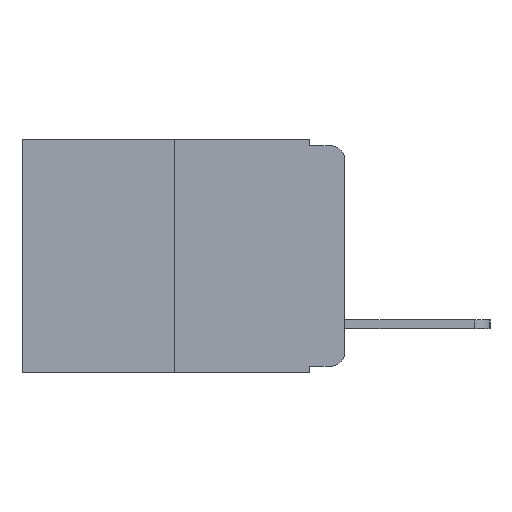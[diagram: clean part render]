
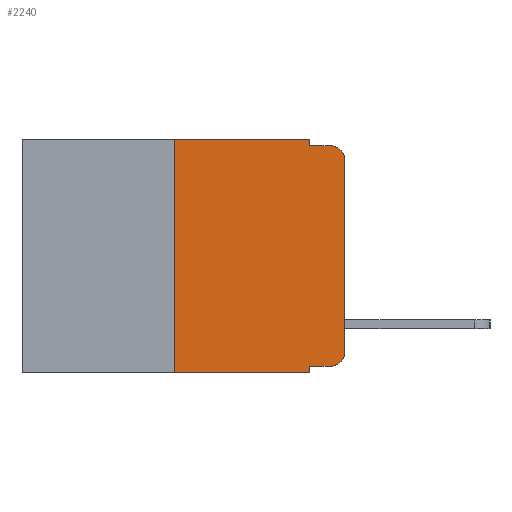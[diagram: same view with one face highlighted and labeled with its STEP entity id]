
A CAD part, left-side view. The second image highlights one B-rep face of the part: STEP entity #2240.
In plain terms, the highlighted planar face has unit normal (-1, 0, 0).
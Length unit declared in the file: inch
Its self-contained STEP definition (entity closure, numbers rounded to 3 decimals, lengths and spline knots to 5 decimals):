
#42 = CARTESIAN_POINT ( 'NONE',  ( 0., 0.051, -0.01 ) ) ;
#947 = LINE ( 'NONE', #42, #8974 ) ;
#1039 = CARTESIAN_POINT ( 'NONE',  ( 0., 0.473, -0.343 ) ) ;
#1554 = CARTESIAN_POINT ( 'NONE',  ( 0., 0.051, 0. ) ) ;
#1829 = DIRECTION ( 'NONE',  ( -1., 0., 0. ) ) ;
#1898 = CARTESIAN_POINT ( 'NONE',  ( 0., 0.051, -0.01 ) ) ;
#2240 = ADVANCED_FACE ( 'NONE', ( #6788 ), #15060, .F. ) ;
#2954 = VERTEX_POINT ( 'NONE', #7508 ) ;
#3170 = DIRECTION ( 'NONE',  ( 0., 0., -1. ) ) ;
#3382 = EDGE_CURVE ( 'NONE', #13404, #9076, #7273, .T. ) ;
#3409 = AXIS2_PLACEMENT_3D ( 'NONE', #17001, #5361, #14315 ) ;
#3905 = AXIS2_PLACEMENT_3D ( 'NONE', #11383, #1829, #12940 ) ;
#3995 = VECTOR ( 'NONE', #15315, 39.37008 ) ;
#4222 = VERTEX_POINT ( 'NONE', #12946 ) ;
#4540 = ORIENTED_EDGE ( 'NONE', *, *, #11252, .F. ) ;
#4566 = VERTEX_POINT ( 'NONE', #19876 ) ;
#4874 = DIRECTION ( 'NONE',  ( -1., 0., 0. ) ) ;
#4983 = LINE ( 'NONE', #13770, #3995 ) ;
#5032 = ORIENTED_EDGE ( 'NONE', *, *, #9139, .T. ) ;
#5293 = CARTESIAN_POINT ( 'NONE',  ( 0., 0.02, -0.333 ) ) ;
#5361 = DIRECTION ( 'NONE',  ( 1., 0., 0. ) ) ;
#5432 = VECTOR ( 'NONE', #17226, 39.37008 ) ;
#5838 = EDGE_LOOP ( 'NONE', ( #10028, #14164, #11028, #15128, #19176, #7824, #16082, #4540, #12964, #5032 ) ) ;
#5956 = CARTESIAN_POINT ( 'NONE',  ( 0., 0.25, -0.343 ) ) ;
#6084 = VERTEX_POINT ( 'NONE', #1898 ) ;
#6182 = VECTOR ( 'NONE', #19517, 39.37008 ) ;
#6704 = LINE ( 'NONE', #14941, #6182 ) ;
#6707 = EDGE_CURVE ( 'NONE', #2954, #20347, #14708, .T. ) ;
#6788 = FACE_OUTER_BOUND ( 'NONE', #5838, .T. ) ;
#7054 = LINE ( 'NONE', #15911, #11249 ) ;
#7237 = VECTOR ( 'NONE', #13001, 39.37008 ) ;
#7273 = LINE ( 'NONE', #1039, #15087 ) ;
#7508 = CARTESIAN_POINT ( 'NONE',  ( 0., 0., -0.03 ) ) ;
#7740 = LINE ( 'NONE', #11431, #7237 ) ;
#7824 = ORIENTED_EDGE ( 'NONE', *, *, #11364, .F. ) ;
#8486 = CARTESIAN_POINT ( 'NONE',  ( 0., 0.051, -0.333 ) ) ;
#8608 = DIRECTION ( 'NONE',  ( 0., -1., 0. ) ) ;
#8974 = VECTOR ( 'NONE', #13075, 39.37008 ) ;
#9076 = VERTEX_POINT ( 'NONE', #14132 ) ;
#9139 = EDGE_CURVE ( 'NONE', #10230, #4222, #16585, .T. ) ;
#9927 = VERTEX_POINT ( 'NONE', #15540 ) ;
#10028 = ORIENTED_EDGE ( 'NONE', *, *, #18580, .T. ) ;
#10116 = CARTESIAN_POINT ( 'NONE',  ( 0., 0.02, -0.01 ) ) ;
#10230 = VERTEX_POINT ( 'NONE', #5293 ) ;
#10455 = EDGE_CURVE ( 'NONE', #9927, #6084, #4983, .T. ) ;
#10701 = LINE ( 'NONE', #1554, #14813 ) ;
#11028 = ORIENTED_EDGE ( 'NONE', *, *, #17836, .F. ) ;
#11249 = VECTOR ( 'NONE', #12877, 39.37008 ) ;
#11252 = EDGE_CURVE ( 'NONE', #18482, #9076, #10701, .T. ) ;
#11364 = EDGE_CURVE ( 'NONE', #13404, #4566, #7740, .T. ) ;
#11383 = CARTESIAN_POINT ( 'NONE',  ( 0., 0.02, -0.03 ) ) ;
#11431 = CARTESIAN_POINT ( 'NONE',  ( 0., 0.25, 0. ) ) ;
#12277 = EDGE_CURVE ( 'NONE', #18482, #10230, #15265, .T. ) ;
#12877 = DIRECTION ( 'NONE',  ( 0., -1., 0. ) ) ;
#12940 = DIRECTION ( 'NONE',  ( 0., 0., -1. ) ) ;
#12946 = CARTESIAN_POINT ( 'NONE',  ( 0., 0., -0.313 ) ) ;
#12964 = ORIENTED_EDGE ( 'NONE', *, *, #12277, .T. ) ;
#13001 = DIRECTION ( 'NONE',  ( 0., 0., 1. ) ) ;
#13075 = DIRECTION ( 'NONE',  ( 0., -1., 0. ) ) ;
#13404 = VERTEX_POINT ( 'NONE', #5956 ) ;
#13770 = CARTESIAN_POINT ( 'NONE',  ( 0., 0.051, 0. ) ) ;
#14132 = CARTESIAN_POINT ( 'NONE',  ( 0., 0.051, -0.343 ) ) ;
#14164 = ORIENTED_EDGE ( 'NONE', *, *, #6707, .T. ) ;
#14200 = CARTESIAN_POINT ( 'NONE',  ( 0., 0.051, -0.333 ) ) ;
#14315 = DIRECTION ( 'NONE',  ( 0., 0., -1. ) ) ;
#14333 = CARTESIAN_POINT ( 'NONE',  ( 0., 0.02, -0.313 ) ) ;
#14708 = CIRCLE ( 'NONE', #3905, 0.02 ) ;
#14813 = VECTOR ( 'NONE', #3170, 39.37008 ) ;
#14941 = CARTESIAN_POINT ( 'NONE',  ( 0., 0., 0. ) ) ;
#15060 = PLANE ( 'NONE',  #3409 ) ;
#15087 = VECTOR ( 'NONE', #8608, 39.37008 ) ;
#15128 = ORIENTED_EDGE ( 'NONE', *, *, #10455, .F. ) ;
#15265 = LINE ( 'NONE', #14200, #5432 ) ;
#15315 = DIRECTION ( 'NONE',  ( 0., 0., -1. ) ) ;
#15536 = AXIS2_PLACEMENT_3D ( 'NONE', #14333, #4874, #15867 ) ;
#15540 = CARTESIAN_POINT ( 'NONE',  ( 0., 0.051, 0. ) ) ;
#15867 = DIRECTION ( 'NONE',  ( 0., 0., -1. ) ) ;
#15911 = CARTESIAN_POINT ( 'NONE',  ( 0., 0.473, 0. ) ) ;
#16082 = ORIENTED_EDGE ( 'NONE', *, *, #3382, .T. ) ;
#16585 = CIRCLE ( 'NONE', #15536, 0.02 ) ;
#16666 = EDGE_CURVE ( 'NONE', #4566, #9927, #7054, .T. ) ;
#17001 = CARTESIAN_POINT ( 'NONE',  ( 0., 0.473, 0. ) ) ;
#17226 = DIRECTION ( 'NONE',  ( 0., -1., 0. ) ) ;
#17836 = EDGE_CURVE ( 'NONE', #6084, #20347, #947, .T. ) ;
#18482 = VERTEX_POINT ( 'NONE', #8486 ) ;
#18580 = EDGE_CURVE ( 'NONE', #4222, #2954, #6704, .T. ) ;
#19176 = ORIENTED_EDGE ( 'NONE', *, *, #16666, .F. ) ;
#19517 = DIRECTION ( 'NONE',  ( 0., 0., 1. ) ) ;
#19876 = CARTESIAN_POINT ( 'NONE',  ( 0., 0.25, 0. ) ) ;
#20347 = VERTEX_POINT ( 'NONE', #10116 ) ;
